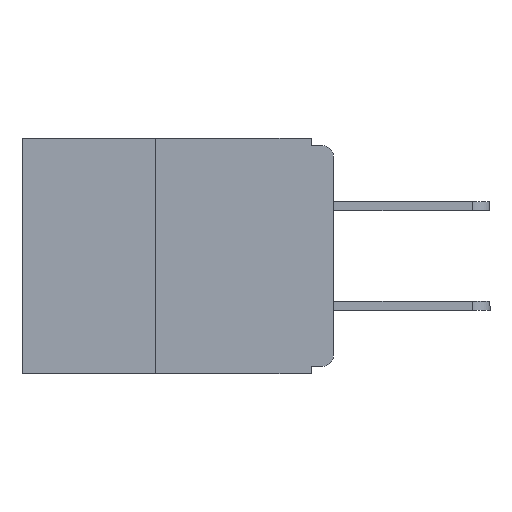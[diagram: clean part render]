
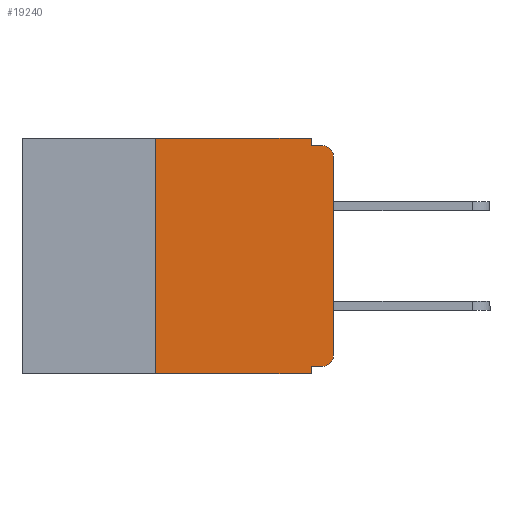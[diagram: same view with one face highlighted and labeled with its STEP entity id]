
A CAD part, left-side view. The second image highlights one B-rep face of the part: STEP entity #19240.
In plain terms, the highlighted planar face has unit normal (-1, 0, 0).
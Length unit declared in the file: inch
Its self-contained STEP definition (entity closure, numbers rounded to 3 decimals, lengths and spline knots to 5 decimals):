
#181 = DIRECTION ( 'NONE',  ( 0., 0., -1. ) ) ;
#466 = VECTOR ( 'NONE', #10628, 39.37008 ) ;
#477 = ORIENTED_EDGE ( 'NONE', *, *, #11605, .F. ) ;
#506 = VERTEX_POINT ( 'NONE', #10574 ) ;
#523 = DIRECTION ( 'NONE',  ( 0., -1., 0. ) ) ;
#911 = CARTESIAN_POINT ( 'NONE',  ( 0., 0., -0.01 ) ) ;
#936 = EDGE_CURVE ( 'NONE', #506, #2593, #8268, .T. ) ;
#1083 = LINE ( 'NONE', #17650, #466 ) ;
#1181 = DIRECTION ( 'NONE',  ( 1., 0., 0. ) ) ;
#1371 = FACE_OUTER_BOUND ( 'NONE', #22863, .T. ) ;
#1458 = CARTESIAN_POINT ( 'NONE',  ( 0., 0.031, -0.32 ) ) ;
#1507 = VECTOR ( 'NONE', #17020, 39.37008 ) ;
#1785 = DIRECTION ( 'NONE',  ( 0., 1., 0. ) ) ;
#2593 = VERTEX_POINT ( 'NONE', #18399 ) ;
#3132 = CARTESIAN_POINT ( 'NONE',  ( 0., 0.031, -0.33 ) ) ;
#3186 = CARTESIAN_POINT ( 'NONE',  ( 0., 0.015, -0.01 ) ) ;
#3304 = ORIENTED_EDGE ( 'NONE', *, *, #17839, .F. ) ;
#3643 = CARTESIAN_POINT ( 'NONE',  ( 0., 0., -0.025 ) ) ;
#3815 = AXIS2_PLACEMENT_3D ( 'NONE', #20040, #20017, #19942 ) ;
#3822 = CARTESIAN_POINT ( 'NONE',  ( 0., 0.25, -0.33 ) ) ;
#4233 = ORIENTED_EDGE ( 'NONE', *, *, #14959, .F. ) ;
#4235 = CARTESIAN_POINT ( 'NONE',  ( 0., 0.437, -0.33 ) ) ;
#4408 = EDGE_CURVE ( 'NONE', #10290, #19923, #6703, .T. ) ;
#4467 = ORIENTED_EDGE ( 'NONE', *, *, #14020, .T. ) ;
#4651 = DIRECTION ( 'NONE',  ( 0., -1., 0. ) ) ;
#4686 = LINE ( 'NONE', #9586, #18176 ) ;
#4707 = CARTESIAN_POINT ( 'NONE',  ( 0., 0.437, 0. ) ) ;
#5065 = ORIENTED_EDGE ( 'NONE', *, *, #7647, .F. ) ;
#5388 = VERTEX_POINT ( 'NONE', #21781 ) ;
#5436 = AXIS2_PLACEMENT_3D ( 'NONE', #21463, #11143, #181 ) ;
#5849 = CARTESIAN_POINT ( 'NONE',  ( 0., 0.015, -0.32 ) ) ;
#6644 = VERTEX_POINT ( 'NONE', #11397 ) ;
#6703 = CIRCLE ( 'NONE', #3815, 0.015 ) ;
#6811 = VECTOR ( 'NONE', #523, 39.37008 ) ;
#7606 = VERTEX_POINT ( 'NONE', #1458 ) ;
#7647 = EDGE_CURVE ( 'NONE', #21021, #19923, #21221, .T. ) ;
#7908 = CIRCLE ( 'NONE', #5436, 0.015 ) ;
#8070 = VECTOR ( 'NONE', #1785, 39.37008 ) ;
#8268 = LINE ( 'NONE', #4235, #12417 ) ;
#8411 = CARTESIAN_POINT ( 'NONE',  ( 0., 0.031, -0.01 ) ) ;
#8639 = AXIS2_PLACEMENT_3D ( 'NONE', #10252, #1181, #13827 ) ;
#8679 = LINE ( 'NONE', #4707, #1507 ) ;
#9562 = VERTEX_POINT ( 'NONE', #11900 ) ;
#9586 = CARTESIAN_POINT ( 'NONE',  ( 0., 0.031, 0. ) ) ;
#10020 = ORIENTED_EDGE ( 'NONE', *, *, #21876, .T. ) ;
#10180 = LINE ( 'NONE', #3822, #11863 ) ;
#10252 = CARTESIAN_POINT ( 'NONE',  ( 0., 0.437, 0. ) ) ;
#10290 = VERTEX_POINT ( 'NONE', #3643 ) ;
#10526 = ORIENTED_EDGE ( 'NONE', *, *, #19445, .F. ) ;
#10574 = CARTESIAN_POINT ( 'NONE',  ( 0., 0.25, -0.33 ) ) ;
#10628 = DIRECTION ( 'NONE',  ( 0., 0., 1. ) ) ;
#11143 = DIRECTION ( 'NONE',  ( -1., 0., 0. ) ) ;
#11397 = CARTESIAN_POINT ( 'NONE',  ( 0., 0.031, 0. ) ) ;
#11605 = EDGE_CURVE ( 'NONE', #5388, #6644, #8679, .T. ) ;
#11863 = VECTOR ( 'NONE', #16158, 39.37008 ) ;
#11900 = CARTESIAN_POINT ( 'NONE',  ( 0., 0., -0.305 ) ) ;
#12056 = DIRECTION ( 'NONE',  ( 0., 0., -1. ) ) ;
#12417 = VECTOR ( 'NONE', #4651, 39.37008 ) ;
#12496 = ORIENTED_EDGE ( 'NONE', *, *, #4408, .T. ) ;
#13827 = DIRECTION ( 'NONE',  ( 0., 0., -1. ) ) ;
#14020 = EDGE_CURVE ( 'NONE', #9562, #10290, #1083, .T. ) ;
#14458 = CARTESIAN_POINT ( 'NONE',  ( 0., 0., -0.32 ) ) ;
#14630 = VECTOR ( 'NONE', #12056, 39.37008 ) ;
#14934 = DIRECTION ( 'NONE',  ( 0., 0., -1. ) ) ;
#14959 = EDGE_CURVE ( 'NONE', #6644, #21021, #4686, .T. ) ;
#16158 = DIRECTION ( 'NONE',  ( 0., 0., 1. ) ) ;
#16693 = VERTEX_POINT ( 'NONE', #5849 ) ;
#17020 = DIRECTION ( 'NONE',  ( 0., -1., 0. ) ) ;
#17650 = CARTESIAN_POINT ( 'NONE',  ( 0., 0., 0. ) ) ;
#17839 = EDGE_CURVE ( 'NONE', #16693, #7606, #22396, .T. ) ;
#18176 = VECTOR ( 'NONE', #14934, 39.37008 ) ;
#18399 = CARTESIAN_POINT ( 'NONE',  ( 0., 0.031, -0.33 ) ) ;
#18521 = ORIENTED_EDGE ( 'NONE', *, *, #936, .T. ) ;
#19240 = ADVANCED_FACE ( 'NONE', ( #1371 ), #22306, .F. ) ;
#19249 = EDGE_CURVE ( 'NONE', #7606, #2593, #19742, .T. ) ;
#19445 = EDGE_CURVE ( 'NONE', #506, #5388, #10180, .T. ) ;
#19742 = LINE ( 'NONE', #3132, #14630 ) ;
#19923 = VERTEX_POINT ( 'NONE', #3186 ) ;
#19942 = DIRECTION ( 'NONE',  ( 0., 0., -1. ) ) ;
#20017 = DIRECTION ( 'NONE',  ( -1., 0., 0. ) ) ;
#20040 = CARTESIAN_POINT ( 'NONE',  ( 0., 0.015, -0.025 ) ) ;
#21021 = VERTEX_POINT ( 'NONE', #8411 ) ;
#21221 = LINE ( 'NONE', #911, #6811 ) ;
#21463 = CARTESIAN_POINT ( 'NONE',  ( 0., 0.015, -0.305 ) ) ;
#21781 = CARTESIAN_POINT ( 'NONE',  ( 0., 0.25, 0. ) ) ;
#21876 = EDGE_CURVE ( 'NONE', #16693, #9562, #7908, .T. ) ;
#22145 = ORIENTED_EDGE ( 'NONE', *, *, #19249, .F. ) ;
#22306 = PLANE ( 'NONE',  #8639 ) ;
#22396 = LINE ( 'NONE', #14458, #8070 ) ;
#22863 = EDGE_LOOP ( 'NONE', ( #4467, #12496, #5065, #4233, #477, #10526, #18521, #22145, #3304, #10020 ) ) ;
